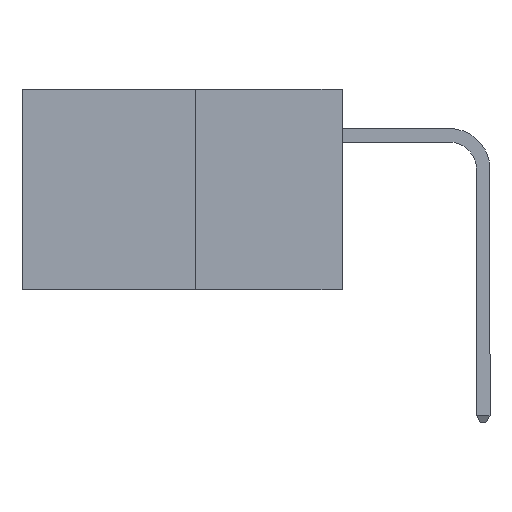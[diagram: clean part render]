
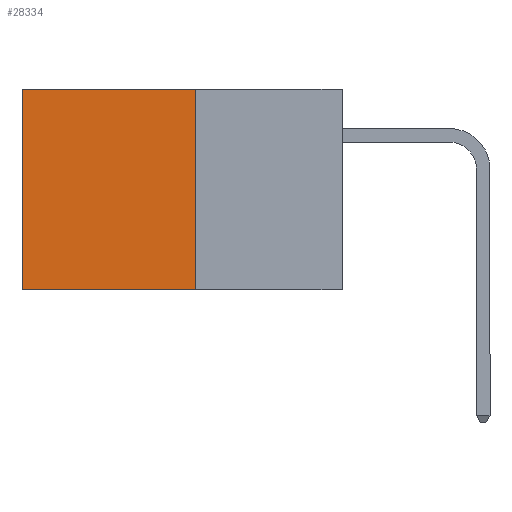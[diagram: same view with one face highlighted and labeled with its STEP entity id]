
A CAD part, left-side view. The second image highlights one B-rep face of the part: STEP entity #28334.
In plain terms, the highlighted planar face has unit normal (-1, 0, 0).
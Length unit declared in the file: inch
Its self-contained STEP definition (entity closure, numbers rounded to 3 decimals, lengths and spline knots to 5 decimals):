
#1689 = VECTOR ( 'NONE', #10573, 39.37008 ) ;
#1708 = ORIENTED_EDGE ( 'NONE', *, *, #10789, .F. ) ;
#1746 = ORIENTED_EDGE ( 'NONE', *, *, #6191, .T. ) ;
#2343 = CARTESIAN_POINT ( 'NONE',  ( 0.277, 0.59, 0. ) ) ;
#2890 = VERTEX_POINT ( 'NONE', #11091 ) ;
#6191 = EDGE_CURVE ( 'NONE', #8415, #21912, #6445, .T. ) ;
#6445 = LINE ( 'NONE', #15985, #27486 ) ;
#6775 = AXIS2_PLACEMENT_3D ( 'NONE', #18102, #11623, #26733 ) ;
#6809 = EDGE_CURVE ( 'NONE', #21912, #17991, #11274, .T. ) ;
#7850 = LINE ( 'NONE', #28542, #8566 ) ;
#8212 = CARTESIAN_POINT ( 'NONE',  ( 0.277, 0.27, 0. ) ) ;
#8410 = CARTESIAN_POINT ( 'NONE',  ( 0.277, 0.27, -0.37 ) ) ;
#8415 = VERTEX_POINT ( 'NONE', #8212 ) ;
#8566 = VECTOR ( 'NONE', #13556, 39.37008 ) ;
#10275 = EDGE_CURVE ( 'NONE', #2890, #17991, #7850, .T. ) ;
#10573 = DIRECTION ( 'NONE',  ( 0., 0., -1. ) ) ;
#10608 = VECTOR ( 'NONE', #27227, 39.37008 ) ;
#10789 = EDGE_CURVE ( 'NONE', #8415, #2890, #19426, .T. ) ;
#11091 = CARTESIAN_POINT ( 'NONE',  ( 0.277, 0.27, -0.37 ) ) ;
#11274 = LINE ( 'NONE', #27133, #10608 ) ;
#11486 = FACE_OUTER_BOUND ( 'NONE', #13231, .T. ) ;
#11623 = DIRECTION ( 'NONE',  ( 1., 0., 0. ) ) ;
#13231 = EDGE_LOOP ( 'NONE', ( #23591, #18830, #1708, #1746 ) ) ;
#13556 = DIRECTION ( 'NONE',  ( 0., 1., 0. ) ) ;
#14142 = CARTESIAN_POINT ( 'NONE',  ( 0.277, 0.59, -0.37 ) ) ;
#15985 = CARTESIAN_POINT ( 'NONE',  ( 0.277, 0.27, 0. ) ) ;
#17991 = VERTEX_POINT ( 'NONE', #14142 ) ;
#18102 = CARTESIAN_POINT ( 'NONE',  ( 0.277, 0.27, -0.37 ) ) ;
#18172 = DIRECTION ( 'NONE',  ( 0., 1., 0. ) ) ;
#18830 = ORIENTED_EDGE ( 'NONE', *, *, #10275, .F. ) ;
#19426 = LINE ( 'NONE', #8410, #1689 ) ;
#21912 = VERTEX_POINT ( 'NONE', #2343 ) ;
#23591 = ORIENTED_EDGE ( 'NONE', *, *, #6809, .T. ) ;
#24631 = PLANE ( 'NONE',  #6775 ) ;
#26733 = DIRECTION ( 'NONE',  ( 0., 0., -1. ) ) ;
#27133 = CARTESIAN_POINT ( 'NONE',  ( 0.277, 0.59, -0.37 ) ) ;
#27227 = DIRECTION ( 'NONE',  ( 0., 0., -1. ) ) ;
#27486 = VECTOR ( 'NONE', #18172, 39.37008 ) ;
#28334 = ADVANCED_FACE ( 'NONE', ( #11486 ), #24631, .F. ) ;
#28542 = CARTESIAN_POINT ( 'NONE',  ( 0.277, 0.27, -0.37 ) ) ;
